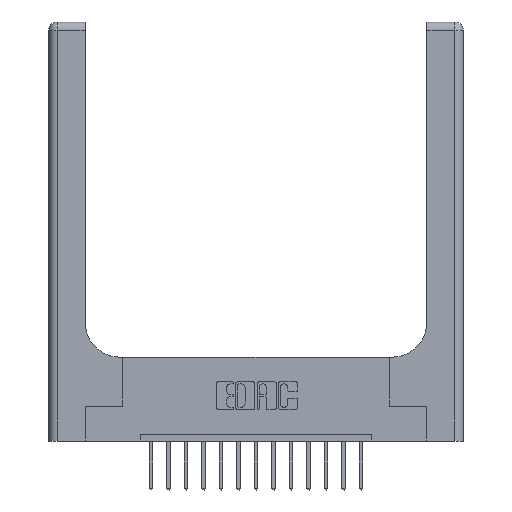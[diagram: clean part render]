
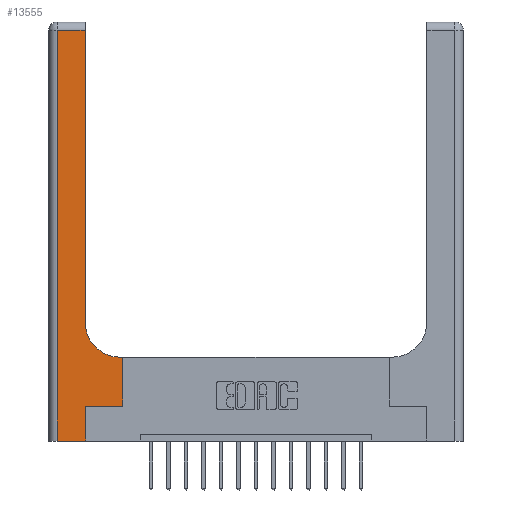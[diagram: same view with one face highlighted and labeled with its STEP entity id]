
A CAD part, top view. The second image highlights one B-rep face of the part: STEP entity #13555.
In plain terms, the highlighted planar face has unit normal (0, 0, 1).
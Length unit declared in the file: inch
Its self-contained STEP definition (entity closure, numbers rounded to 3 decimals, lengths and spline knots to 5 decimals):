
#84 = DIRECTION ( 'NONE',  ( 0., 0., -1. ) ) ;
#231 = LINE ( 'NONE', #3611, #1653 ) ;
#278 = CARTESIAN_POINT ( 'NONE',  ( 0.265, 0., 0.37 ) ) ;
#871 = DIRECTION ( 'NONE',  ( 0., 1., 0. ) ) ;
#1057 = CARTESIAN_POINT ( 'NONE',  ( 0.528, 0.6, 0.37 ) ) ;
#1095 = ORIENTED_EDGE ( 'NONE', *, *, #9395, .T. ) ;
#1148 = ORIENTED_EDGE ( 'NONE', *, *, #2803, .T. ) ;
#1247 = AXIS2_PLACEMENT_3D ( 'NONE', #12056, #84, #5322 ) ;
#1653 = VECTOR ( 'NONE', #871, 39.37008 ) ;
#1979 = EDGE_CURVE ( 'NONE', #10972, #6322, #16624, .T. ) ;
#2232 = LINE ( 'NONE', #4106, #9118 ) ;
#2248 = VECTOR ( 'NONE', #7610, 39.37008 ) ;
#2270 = DIRECTION ( 'NONE',  ( 0., 1., 0. ) ) ;
#2299 = CARTESIAN_POINT ( 'NONE',  ( 0.51, 0.6, 0.37 ) ) ;
#2517 = VECTOR ( 'NONE', #8981, 39.37008 ) ;
#2803 = EDGE_CURVE ( 'NONE', #6322, #15435, #231, .T. ) ;
#3460 = CARTESIAN_POINT ( 'NONE',  ( 0.06, 0., 0.37 ) ) ;
#3598 = VECTOR ( 'NONE', #2270, 39.37008 ) ;
#3611 = CARTESIAN_POINT ( 'NONE',  ( 0.528, 0.25, 0.37 ) ) ;
#3712 = LINE ( 'NONE', #14215, #2248 ) ;
#3785 = VERTEX_POINT ( 'NONE', #9284 ) ;
#4031 = VERTEX_POINT ( 'NONE', #7433 ) ;
#4106 = CARTESIAN_POINT ( 'NONE',  ( 0.26, 3., 0.37 ) ) ;
#4351 = EDGE_CURVE ( 'NONE', #15198, #8081, #6424, .T. ) ;
#4452 = EDGE_CURVE ( 'NONE', #3785, #4031, #2232, .T. ) ;
#4870 = ORIENTED_EDGE ( 'NONE', *, *, #13718, .T. ) ;
#5055 = ORIENTED_EDGE ( 'NONE', *, *, #13124, .T. ) ;
#5322 = DIRECTION ( 'NONE',  ( 1., 0., 0. ) ) ;
#5359 = CARTESIAN_POINT ( 'NONE',  ( 0.528, 0.25, 0.37 ) ) ;
#5642 = LINE ( 'NONE', #11063, #15793 ) ;
#6214 = VECTOR ( 'NONE', #14655, 39.37008 ) ;
#6322 = VERTEX_POINT ( 'NONE', #5359 ) ;
#6412 = AXIS2_PLACEMENT_3D ( 'NONE', #11850, #17104, #15675 ) ;
#6424 = LINE ( 'NONE', #11937, #6214 ) ;
#7268 = VERTEX_POINT ( 'NONE', #278 ) ;
#7433 = CARTESIAN_POINT ( 'NONE',  ( 0.26, 2.94, 0.37 ) ) ;
#7610 = DIRECTION ( 'NONE',  ( 1., 0., 0. ) ) ;
#8081 = VERTEX_POINT ( 'NONE', #3460 ) ;
#8356 = CARTESIAN_POINT ( 'NONE',  ( 0.26, 0.6, 0.37 ) ) ;
#8430 = CARTESIAN_POINT ( 'NONE',  ( 0.06, 2.94, 0.37 ) ) ;
#8504 = ORIENTED_EDGE ( 'NONE', *, *, #4452, .T. ) ;
#8981 = DIRECTION ( 'NONE',  ( 1., 0., 0. ) ) ;
#9118 = VECTOR ( 'NONE', #9231, 39.37008 ) ;
#9127 = DIRECTION ( 'NONE',  ( -1., 0., 0. ) ) ;
#9231 = DIRECTION ( 'NONE',  ( 0., 1., 0. ) ) ;
#9284 = CARTESIAN_POINT ( 'NONE',  ( 0.26, 0.85, 0.37 ) ) ;
#9395 = EDGE_CURVE ( 'NONE', #4031, #15198, #5642, .T. ) ;
#10378 = EDGE_CURVE ( 'NONE', #8081, #7268, #3712, .T. ) ;
#10972 = VERTEX_POINT ( 'NONE', #13965 ) ;
#11063 = CARTESIAN_POINT ( 'NONE',  ( 0., 2.94, 0.37 ) ) ;
#11282 = VECTOR ( 'NONE', #9127, 39.37008 ) ;
#11850 = CARTESIAN_POINT ( 'NONE',  ( 0., 3., 0.37 ) ) ;
#11937 = CARTESIAN_POINT ( 'NONE',  ( 0.06, 3., 0.37 ) ) ;
#11953 = CIRCLE ( 'NONE', #1247, 0.25 ) ;
#12056 = CARTESIAN_POINT ( 'NONE',  ( 0.51, 0.85, 0.37 ) ) ;
#12527 = LINE ( 'NONE', #8356, #11282 ) ;
#12535 = VERTEX_POINT ( 'NONE', #2299 ) ;
#12556 = CARTESIAN_POINT ( 'NONE',  ( 0.265, 0., 0.37 ) ) ;
#12757 = ORIENTED_EDGE ( 'NONE', *, *, #10378, .T. ) ;
#12787 = ORIENTED_EDGE ( 'NONE', *, *, #1979, .T. ) ;
#13124 = EDGE_CURVE ( 'NONE', #12535, #3785, #11953, .T. ) ;
#13195 = CARTESIAN_POINT ( 'NONE',  ( 0.265, 0.25, 0.37 ) ) ;
#13555 = ADVANCED_FACE ( 'NONE', ( #14825 ), #14061, .F. ) ;
#13718 = EDGE_CURVE ( 'NONE', #7268, #10972, #14412, .T. ) ;
#13965 = CARTESIAN_POINT ( 'NONE',  ( 0.265, 0.25, 0.37 ) ) ;
#14061 = PLANE ( 'NONE',  #6412 ) ;
#14215 = CARTESIAN_POINT ( 'NONE',  ( 0., 0., 0.37 ) ) ;
#14223 = ORIENTED_EDGE ( 'NONE', *, *, #16455, .T. ) ;
#14412 = LINE ( 'NONE', #12556, #3598 ) ;
#14655 = DIRECTION ( 'NONE',  ( 0., -1., 0. ) ) ;
#14825 = FACE_OUTER_BOUND ( 'NONE', #15403, .T. ) ;
#15150 = DIRECTION ( 'NONE',  ( -1., 0., 0. ) ) ;
#15198 = VERTEX_POINT ( 'NONE', #8430 ) ;
#15403 = EDGE_LOOP ( 'NONE', ( #8504, #1095, #16446, #12757, #4870, #12787, #1148, #14223, #5055 ) ) ;
#15435 = VERTEX_POINT ( 'NONE', #1057 ) ;
#15675 = DIRECTION ( 'NONE',  ( -1., 0., 0. ) ) ;
#15793 = VECTOR ( 'NONE', #15150, 39.37008 ) ;
#16446 = ORIENTED_EDGE ( 'NONE', *, *, #4351, .T. ) ;
#16455 = EDGE_CURVE ( 'NONE', #15435, #12535, #12527, .T. ) ;
#16624 = LINE ( 'NONE', #13195, #2517 ) ;
#17104 = DIRECTION ( 'NONE',  ( 0., 0., -1. ) ) ;
